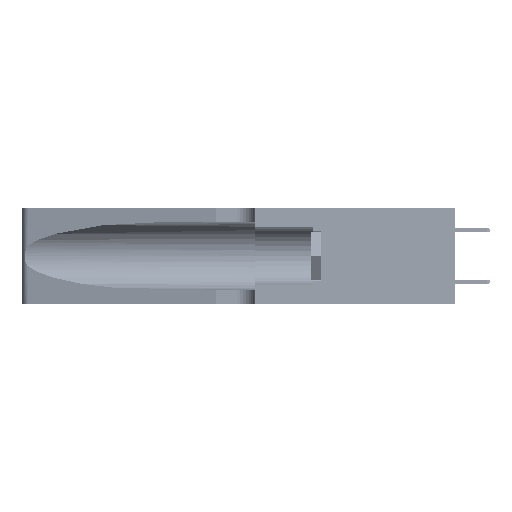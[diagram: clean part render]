
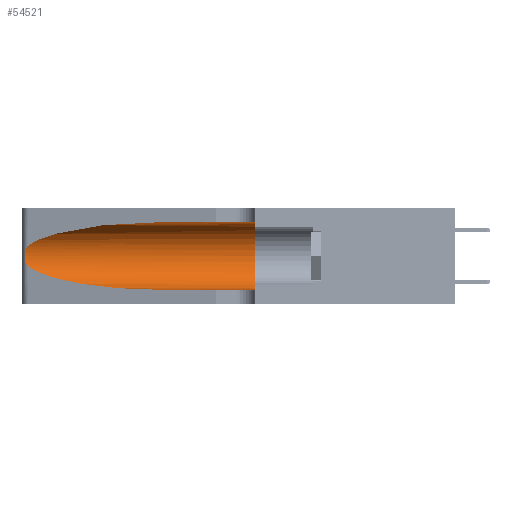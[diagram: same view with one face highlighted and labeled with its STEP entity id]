
A CAD part, left-side view. The second image highlights one B-rep face of the part: STEP entity #54521.
In plain terms, the highlighted cylindrical face has radius 3.308 mm (diameter 6.617 mm), a partial arc.
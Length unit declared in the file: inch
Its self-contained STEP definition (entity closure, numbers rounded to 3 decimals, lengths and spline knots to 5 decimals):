
#329 = CARTESIAN_POINT ( 'NONE',  ( 0.18966, 0.96281, 0.05475 ) ) ;
#1110 = CARTESIAN_POINT ( 'NONE',  ( 0.18966, 0.96281, 0.31525 ) ) ;
#1162 = CARTESIAN_POINT ( 'NONE',  ( 0.1305, 1.61858, 0.185 ) ) ;
#2459 = CARTESIAN_POINT ( 'NONE',  ( 0.1305, 0.72297, 0.05475 ) ) ;
#2464 = CARTESIAN_POINT ( 'NONE',  ( 0.25639, 1.23186, 0.15144 ) ) ;
#4136 = CARTESIAN_POINT ( 'NONE',  ( 0.1305, 1.61858, 0.31525 ) ) ;
#4781 = CARTESIAN_POINT ( 'NONE',  ( 0.25487, 1.22718, 0.14631 ) ) ;
#5465 = ORIENTED_EDGE ( 'NONE', *, *, #38208, .T. ) ;
#6381 = CARTESIAN_POINT ( 'NONE',  ( 0.25555, 1.22993, 0.14849 ) ) ;
#7841 =( BOUNDED_CURVE ( )  B_SPLINE_CURVE ( 3, ( #4781, #50611, #329, #50877 ),
 .UNSPECIFIED., .F., .T. ) 
 B_SPLINE_CURVE_WITH_KNOTS ( ( 4, 4 ),
 ( 3.44316, 4.71239 ),
 .UNSPECIFIED. ) 
 CURVE ( )  GEOMETRIC_REPRESENTATION_ITEM ( )  RATIONAL_B_SPLINE_CURVE ( ( 1., 0.87, 0.87, 1. ) ) 
 REPRESENTATION_ITEM ( '' )  );
#9738 = CARTESIAN_POINT ( 'NONE',  ( 0.25639, 1.23184, 0.21858 ) ) ;
#10273 = CARTESIAN_POINT ( 'NONE',  ( 0.25856, 1.23593, 0.16098 ) ) ;
#11358 = CARTESIAN_POINT ( 'NONE',  ( 0.25487, 1.22718, 0.14631 ) ) ;
#11549 = DIRECTION ( 'NONE',  ( 0., 0., 1. ) ) ;
#12791 = VERTEX_POINT ( 'NONE', #46196 ) ;
#13341 = CARTESIAN_POINT ( 'NONE',  ( 0.26018, 1.23835, 0.19895 ) ) ;
#14094 = EDGE_CURVE ( 'NONE', #42497, #33226, #7841, .T. ) ;
#15710 = CARTESIAN_POINT ( 'NONE',  ( 0.1305, 0.35, 0.185 ) ) ;
#15902 = ORIENTED_EDGE ( 'NONE', *, *, #49090, .F. ) ;
#16946 = LINE ( 'NONE', #4136, #39959 ) ;
#17259 = VERTEX_POINT ( 'NONE', #53023 ) ;
#17481 = VERTEX_POINT ( 'NONE', #19717 ) ;
#17508 = CARTESIAN_POINT ( 'NONE',  ( 0.25854, 1.2359, 0.20912 ) ) ;
#17516 = CARTESIAN_POINT ( 'NONE',  ( 0.1305, 0.72297, 0.31525 ) ) ;
#19717 = CARTESIAN_POINT ( 'NONE',  ( 0.1305, 0.72297, 0.31525 ) ) ;
#21117 = DIRECTION ( 'NONE',  ( 0., -1., 0. ) ) ;
#21683 = CARTESIAN_POINT ( 'NONE',  ( 0.25555, 1.22994, 0.2215 ) ) ;
#21962 = CARTESIAN_POINT ( 'NONE',  ( 0.26017, 1.23833, 0.17102 ) ) ;
#22094 = ORIENTED_EDGE ( 'NONE', *, *, #34187, .T. ) ;
#23132 = CARTESIAN_POINT ( 'NONE',  ( 0.1305, 0.35, 0.31525 ) ) ;
#24032 = VECTOR ( 'NONE', #45080, 39.37008 ) ;
#24548 = AXIS2_PLACEMENT_3D ( 'NONE', #1162, #51949, #26740 ) ;
#26740 = DIRECTION ( 'NONE',  ( 0., 0., -1. ) ) ;
#30277 = CARTESIAN_POINT ( 'NONE',  ( 0.26075, 1.23896, 0.178 ) ) ;
#33226 = VERTEX_POINT ( 'NONE', #2459 ) ;
#33877 = VERTEX_POINT ( 'NONE', #23132 ) ;
#33937 = ORIENTED_EDGE ( 'NONE', *, *, #14094, .T. ) ;
#34187 = EDGE_CURVE ( 'NONE', #17481, #17259, #52076, .T. ) ;
#34452 = CARTESIAN_POINT ( 'NONE',  ( 0.2373, 1.15595, 0.28018 ) ) ;
#34719 = CARTESIAN_POINT ( 'NONE',  ( 0.26075, 1.23896, 0.19203 ) ) ;
#35023 = B_SPLINE_CURVE_WITH_KNOTS ( 'NONE', 3,
 ( #47744, #21683, #9738, #38596, #17508, #13341, #34719, #30277, #21962, #10273, #35825, #2464, #6381, #11358 ),
 .UNSPECIFIED., .F., .F.,
 ( 4, 2, 2, 2, 2, 2, 4 ),
 ( 0., 0.00027, 0.00053, 0.00107, 0.0016, 0.00187, 0.00214 ),
 .UNSPECIFIED. ) ;
#35055 = CYLINDRICAL_SURFACE ( 'NONE', #24548, 0.13025 ) ;
#35825 = CARTESIAN_POINT ( 'NONE',  ( 0.25789, 1.23486, 0.15765 ) ) ;
#36095 = CARTESIAN_POINT ( 'NONE',  ( 0.25487, 1.22718, 0.14631 ) ) ;
#38208 = EDGE_CURVE ( 'NONE', #33226, #12791, #40631, .T. ) ;
#38596 = CARTESIAN_POINT ( 'NONE',  ( 0.25787, 1.23484, 0.2124 ) ) ;
#38690 = ORIENTED_EDGE ( 'NONE', *, *, #53768, .F. ) ;
#39959 = VECTOR ( 'NONE', #21117, 39.37008 ) ;
#40370 = AXIS2_PLACEMENT_3D ( 'NONE', #15710, #53199, #11549 ) ;
#40631 = LINE ( 'NONE', #53413, #24032 ) ;
#42134 = CIRCLE ( 'NONE', #40370, 0.13025 ) ;
#42346 = EDGE_CURVE ( 'NONE', #17259, #42497, #35023, .T. ) ;
#42497 = VERTEX_POINT ( 'NONE', #36095 ) ;
#45080 = DIRECTION ( 'NONE',  ( 0., -1., 0. ) ) ;
#46196 = CARTESIAN_POINT ( 'NONE',  ( 0.1305, 0.35, 0.05475 ) ) ;
#47744 = CARTESIAN_POINT ( 'NONE',  ( 0.25487, 1.22718, 0.22369 ) ) ;
#48040 = ORIENTED_EDGE ( 'NONE', *, *, #42346, .T. ) ;
#49090 = EDGE_CURVE ( 'NONE', #17481, #33877, #16946, .T. ) ;
#50611 = CARTESIAN_POINT ( 'NONE',  ( 0.2373, 1.15595, 0.08982 ) ) ;
#50827 = CARTESIAN_POINT ( 'NONE',  ( 0.25487, 1.22718, 0.22369 ) ) ;
#50877 = CARTESIAN_POINT ( 'NONE',  ( 0.1305, 0.72297, 0.05475 ) ) ;
#51608 = EDGE_LOOP ( 'NONE', ( #22094, #48040, #33937, #5465, #38690, #15902 ) ) ;
#51691 = FACE_OUTER_BOUND ( 'NONE', #51608, .T. ) ;
#51949 = DIRECTION ( 'NONE',  ( 0., -1., 0. ) ) ;
#52076 =( BOUNDED_CURVE ( )  B_SPLINE_CURVE ( 3, ( #17516, #1110, #34452, #50827 ),
 .UNSPECIFIED., .F., .T. ) 
 B_SPLINE_CURVE_WITH_KNOTS ( ( 4, 4 ),
 ( 1.5708, 2.84003 ),
 .UNSPECIFIED. ) 
 CURVE ( )  GEOMETRIC_REPRESENTATION_ITEM ( )  RATIONAL_B_SPLINE_CURVE ( ( 1., 0.87, 0.87, 1. ) ) 
 REPRESENTATION_ITEM ( '' )  );
#53023 = CARTESIAN_POINT ( 'NONE',  ( 0.25487, 1.22718, 0.22369 ) ) ;
#53199 = DIRECTION ( 'NONE',  ( 0., 1., 0. ) ) ;
#53413 = CARTESIAN_POINT ( 'NONE',  ( 0.1305, 1.61858, 0.05475 ) ) ;
#53768 = EDGE_CURVE ( 'NONE', #33877, #12791, #42134, .T. ) ;
#54521 = ADVANCED_FACE ( 'NONE', ( #51691 ), #35055, .F. ) ;
